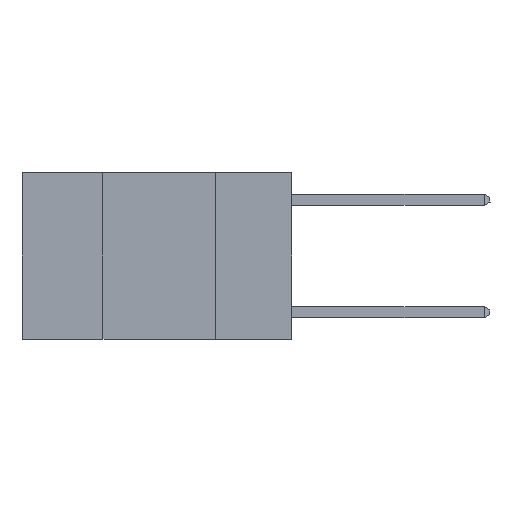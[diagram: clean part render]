
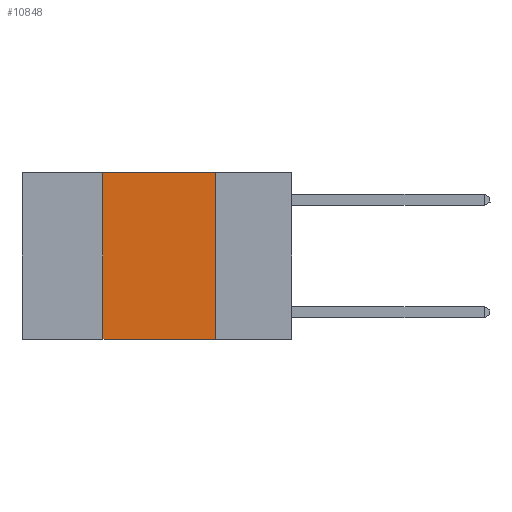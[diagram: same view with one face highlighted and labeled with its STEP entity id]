
A CAD part, left-side view. The second image highlights one B-rep face of the part: STEP entity #10848.
In plain terms, the highlighted planar face has unit normal (-1, 0, 0).
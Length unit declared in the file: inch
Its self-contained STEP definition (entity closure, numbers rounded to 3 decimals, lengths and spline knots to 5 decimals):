
#429 = CARTESIAN_POINT ( 'NONE',  ( 0., 0.6, 0. ) ) ;
#439 = CARTESIAN_POINT ( 'NONE',  ( 0., 0.6, 0. ) ) ;
#855 = EDGE_CURVE ( 'NONE', #11387, #10164, #7907, .T. ) ;
#1137 = EDGE_CURVE ( 'NONE', #11387, #3077, #9493, .T. ) ;
#1387 = CARTESIAN_POINT ( 'NONE',  ( 0., 0.17, -0.37 ) ) ;
#1516 = DIRECTION ( 'NONE',  ( 0., 0., -1. ) ) ;
#1527 = DIRECTION ( 'NONE',  ( 0., -1., 0. ) ) ;
#3077 = VERTEX_POINT ( 'NONE', #12789 ) ;
#4769 = CARTESIAN_POINT ( 'NONE',  ( 0., 0.42, -0.37 ) ) ;
#5148 = VECTOR ( 'NONE', #9327, 39.37008 ) ;
#5713 = PLANE ( 'NONE',  #12116 ) ;
#5902 = ORIENTED_EDGE ( 'NONE', *, *, #8665, .F. ) ;
#6023 = ORIENTED_EDGE ( 'NONE', *, *, #7144, .F. ) ;
#6162 = ORIENTED_EDGE ( 'NONE', *, *, #1137, .F. ) ;
#6224 = ORIENTED_EDGE ( 'NONE', *, *, #855, .T. ) ;
#6382 = VECTOR ( 'NONE', #13105, 39.37008 ) ;
#7144 = EDGE_CURVE ( 'NONE', #3077, #9870, #8001, .T. ) ;
#7277 = FACE_OUTER_BOUND ( 'NONE', #8263, .T. ) ;
#7437 = VECTOR ( 'NONE', #9215, 39.37008 ) ;
#7789 = DIRECTION ( 'NONE',  ( 1., 0., 0. ) ) ;
#7907 = LINE ( 'NONE', #11013, #5148 ) ;
#8001 = LINE ( 'NONE', #439, #12902 ) ;
#8252 = CARTESIAN_POINT ( 'NONE',  ( 0., 0.17, 0. ) ) ;
#8263 = EDGE_LOOP ( 'NONE', ( #5902, #6023, #6162, #6224 ) ) ;
#8665 = EDGE_CURVE ( 'NONE', #9870, #10164, #9090, .T. ) ;
#8892 = CARTESIAN_POINT ( 'NONE',  ( 0., 0.42, 0. ) ) ;
#9090 = LINE ( 'NONE', #8252, #6382 ) ;
#9215 = DIRECTION ( 'NONE',  ( 0., 0., 1. ) ) ;
#9233 = CARTESIAN_POINT ( 'NONE',  ( 0., 0.17, 0. ) ) ;
#9327 = DIRECTION ( 'NONE',  ( 0., -1., 0. ) ) ;
#9493 = LINE ( 'NONE', #8892, #7437 ) ;
#9870 = VERTEX_POINT ( 'NONE', #9233 ) ;
#10164 = VERTEX_POINT ( 'NONE', #1387 ) ;
#10848 = ADVANCED_FACE ( 'NONE', ( #7277 ), #5713, .F. ) ;
#11013 = CARTESIAN_POINT ( 'NONE',  ( 0., 0.6, -0.37 ) ) ;
#11387 = VERTEX_POINT ( 'NONE', #4769 ) ;
#12116 = AXIS2_PLACEMENT_3D ( 'NONE', #429, #7789, #1516 ) ;
#12789 = CARTESIAN_POINT ( 'NONE',  ( 0., 0.42, 0. ) ) ;
#12902 = VECTOR ( 'NONE', #1527, 39.37008 ) ;
#13105 = DIRECTION ( 'NONE',  ( 0., 0., -1. ) ) ;
